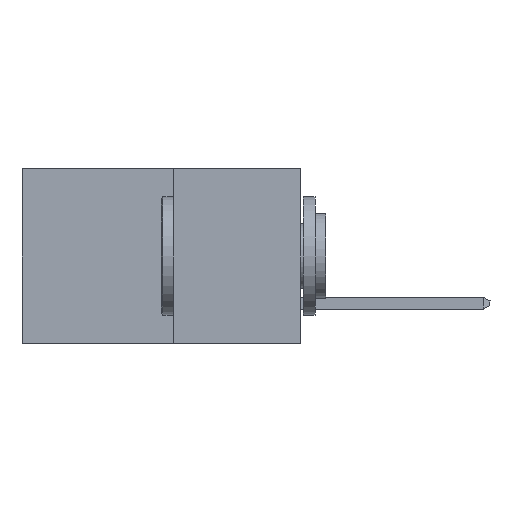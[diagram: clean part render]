
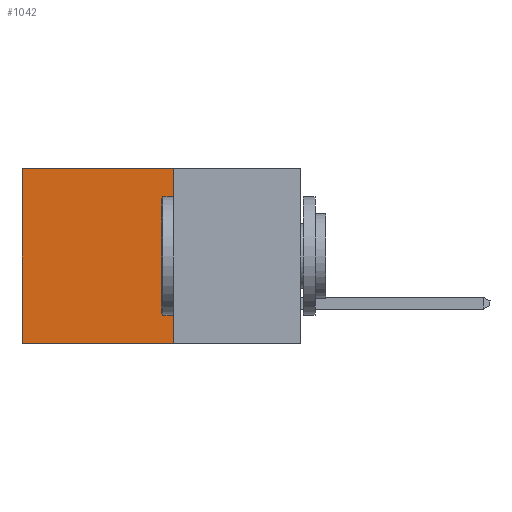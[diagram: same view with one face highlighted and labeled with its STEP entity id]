
A CAD part, left-side view. The second image highlights one B-rep face of the part: STEP entity #1042.
In plain terms, the highlighted planar face has unit normal (-1, 0, 0).
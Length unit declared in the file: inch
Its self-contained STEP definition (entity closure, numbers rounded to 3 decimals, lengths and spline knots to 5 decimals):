
#762 = EDGE_CURVE ( 'NONE', #11387, #10214, #1720, .T. ) ;
#926 = ORIENTED_EDGE ( 'NONE', *, *, #762, .F. ) ;
#1023 = VECTOR ( 'NONE', #1801, 39.37008 ) ;
#1042 = ADVANCED_FACE ( 'NONE', ( #8864 ), #11640, .F. ) ;
#1246 = CARTESIAN_POINT ( 'NONE',  ( 0.277, 0.27, -0.37 ) ) ;
#1396 = VECTOR ( 'NONE', #3245, 39.37008 ) ;
#1618 = CARTESIAN_POINT ( 'NONE',  ( 0.277, 0.59, -0.37 ) ) ;
#1693 = VERTEX_POINT ( 'NONE', #10263 ) ;
#1720 = LINE ( 'NONE', #11109, #1396 ) ;
#1801 = DIRECTION ( 'NONE',  ( 0., 0., -1. ) ) ;
#2201 = CARTESIAN_POINT ( 'NONE',  ( 0.277, 0.27, -0.37 ) ) ;
#2272 = DIRECTION ( 'NONE',  ( 0., 0., -1. ) ) ;
#2504 = VECTOR ( 'NONE', #2272, 39.37008 ) ;
#3127 = ORIENTED_EDGE ( 'NONE', *, *, #4705, .T. ) ;
#3245 = DIRECTION ( 'NONE',  ( 0., 1., 0. ) ) ;
#4185 = ORIENTED_EDGE ( 'NONE', *, *, #10817, .F. ) ;
#4519 = VERTEX_POINT ( 'NONE', #5055 ) ;
#4705 = EDGE_CURVE ( 'NONE', #4519, #10214, #10282, .T. ) ;
#5034 = LINE ( 'NONE', #1246, #2504 ) ;
#5055 = CARTESIAN_POINT ( 'NONE',  ( 0.277, 0.59, 0. ) ) ;
#5059 = DIRECTION ( 'NONE',  ( 1., 0., 0. ) ) ;
#5515 = EDGE_CURVE ( 'NONE', #1693, #4519, #6013, .T. ) ;
#5885 = AXIS2_PLACEMENT_3D ( 'NONE', #10597, #5059, #6918 ) ;
#6013 = LINE ( 'NONE', #7091, #7950 ) ;
#6792 = EDGE_LOOP ( 'NONE', ( #3127, #926, #4185, #9010 ) ) ;
#6918 = DIRECTION ( 'NONE',  ( 0., 0., -1. ) ) ;
#7053 = CARTESIAN_POINT ( 'NONE',  ( 0.277, 0.59, -0.37 ) ) ;
#7091 = CARTESIAN_POINT ( 'NONE',  ( 0.277, 0.27, 0. ) ) ;
#7128 = DIRECTION ( 'NONE',  ( 0., 1., 0. ) ) ;
#7950 = VECTOR ( 'NONE', #7128, 39.37008 ) ;
#8864 = FACE_OUTER_BOUND ( 'NONE', #6792, .T. ) ;
#9010 = ORIENTED_EDGE ( 'NONE', *, *, #5515, .T. ) ;
#10214 = VERTEX_POINT ( 'NONE', #7053 ) ;
#10263 = CARTESIAN_POINT ( 'NONE',  ( 0.277, 0.27, 0. ) ) ;
#10282 = LINE ( 'NONE', #1618, #1023 ) ;
#10597 = CARTESIAN_POINT ( 'NONE',  ( 0.277, 0.27, -0.37 ) ) ;
#10817 = EDGE_CURVE ( 'NONE', #1693, #11387, #5034, .T. ) ;
#11109 = CARTESIAN_POINT ( 'NONE',  ( 0.277, 0.27, -0.37 ) ) ;
#11387 = VERTEX_POINT ( 'NONE', #2201 ) ;
#11640 = PLANE ( 'NONE',  #5885 ) ;
